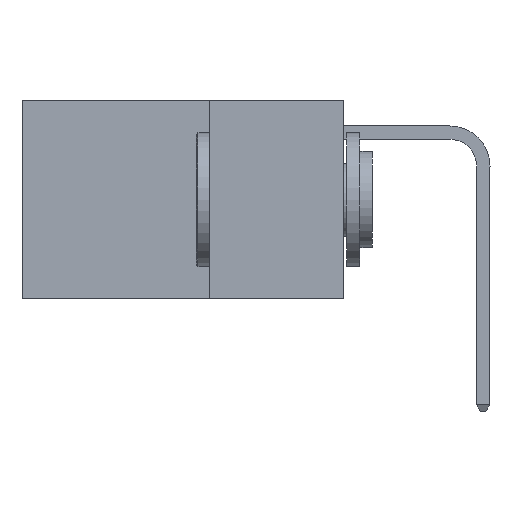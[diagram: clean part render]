
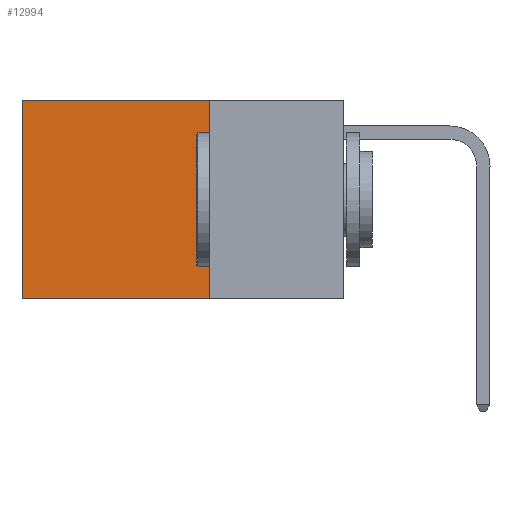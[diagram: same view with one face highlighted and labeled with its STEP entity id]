
A CAD part, left-side view. The second image highlights one B-rep face of the part: STEP entity #12994.
In plain terms, the highlighted planar face has unit normal (-1, 0, 0).
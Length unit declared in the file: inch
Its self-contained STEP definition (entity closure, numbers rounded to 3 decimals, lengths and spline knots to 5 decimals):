
#334 = ORIENTED_EDGE ( 'NONE', *, *, #3849, .F. ) ;
#643 = EDGE_CURVE ( 'NONE', #2777, #13032, #2120, .T. ) ;
#899 = LINE ( 'NONE', #7031, #1021 ) ;
#984 = VERTEX_POINT ( 'NONE', #1322 ) ;
#1021 = VECTOR ( 'NONE', #7048, 39.37008 ) ;
#1322 = CARTESIAN_POINT ( 'NONE',  ( 0.2625, 0.25, -0.37 ) ) ;
#2059 = CARTESIAN_POINT ( 'NONE',  ( 0.2625, 0.6, -0.37 ) ) ;
#2120 = LINE ( 'NONE', #6399, #2365 ) ;
#2365 = VECTOR ( 'NONE', #2660, 39.37008 ) ;
#2374 = CARTESIAN_POINT ( 'NONE',  ( 0.2625, 0.6, 0. ) ) ;
#2496 = DIRECTION ( 'NONE',  ( 0., 0., -1. ) ) ;
#2519 = DIRECTION ( 'NONE',  ( 1., 0., 0. ) ) ;
#2575 = PLANE ( 'NONE',  #12575 ) ;
#2637 = CARTESIAN_POINT ( 'NONE',  ( 0.2625, 0.25, 0. ) ) ;
#2660 = DIRECTION ( 'NONE',  ( 0., 1., 0. ) ) ;
#2777 = VERTEX_POINT ( 'NONE', #4125 ) ;
#3141 = ORIENTED_EDGE ( 'NONE', *, *, #643, .T. ) ;
#3849 = EDGE_CURVE ( 'NONE', #984, #8409, #5495, .T. ) ;
#4125 = CARTESIAN_POINT ( 'NONE',  ( 0.2625, 0.25, 0. ) ) ;
#5096 = DIRECTION ( 'NONE',  ( 0., 0., -1. ) ) ;
#5147 = CARTESIAN_POINT ( 'NONE',  ( 0.2625, 0.6, 0. ) ) ;
#5495 = LINE ( 'NONE', #13450, #5527 ) ;
#5527 = VECTOR ( 'NONE', #13287, 39.37008 ) ;
#6399 = CARTESIAN_POINT ( 'NONE',  ( 0.2625, 0.25, 0. ) ) ;
#7031 = CARTESIAN_POINT ( 'NONE',  ( 0.2625, 0.25, 0. ) ) ;
#7048 = DIRECTION ( 'NONE',  ( 0., 0., -1. ) ) ;
#7624 = ORIENTED_EDGE ( 'NONE', *, *, #12363, .F. ) ;
#7945 = EDGE_LOOP ( 'NONE', ( #13521, #334, #7624, #3141 ) ) ;
#8409 = VERTEX_POINT ( 'NONE', #2059 ) ;
#9260 = VECTOR ( 'NONE', #5096, 39.37008 ) ;
#12157 = FACE_OUTER_BOUND ( 'NONE', #7945, .T. ) ;
#12363 = EDGE_CURVE ( 'NONE', #2777, #984, #899, .T. ) ;
#12575 = AXIS2_PLACEMENT_3D ( 'NONE', #2637, #2519, #2496 ) ;
#12624 = EDGE_CURVE ( 'NONE', #13032, #8409, #13102, .T. ) ;
#12994 = ADVANCED_FACE ( 'NONE', ( #12157 ), #2575, .F. ) ;
#13032 = VERTEX_POINT ( 'NONE', #2374 ) ;
#13102 = LINE ( 'NONE', #5147, #9260 ) ;
#13287 = DIRECTION ( 'NONE',  ( 0., 1., 0. ) ) ;
#13450 = CARTESIAN_POINT ( 'NONE',  ( 0.2625, 0.25, -0.37 ) ) ;
#13521 = ORIENTED_EDGE ( 'NONE', *, *, #12624, .T. ) ;
